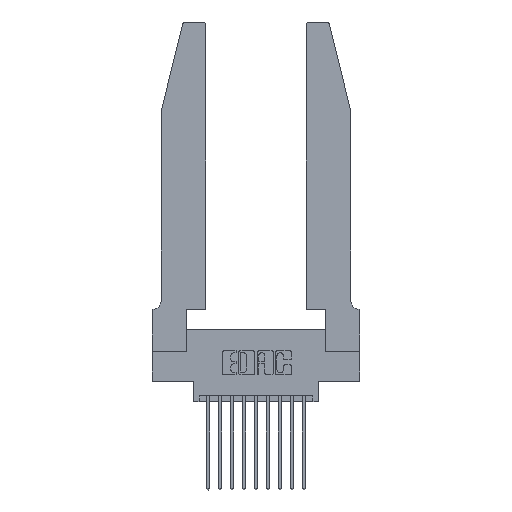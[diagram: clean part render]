
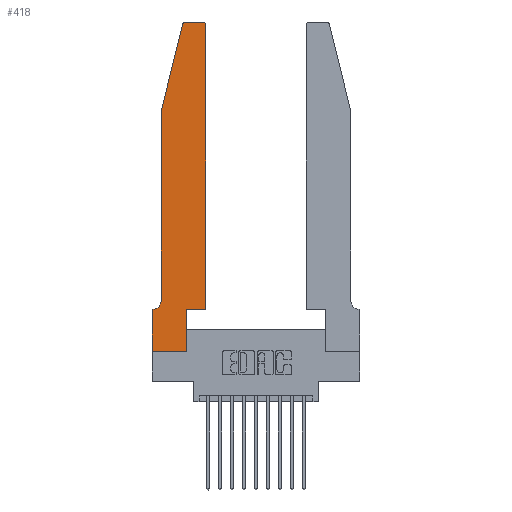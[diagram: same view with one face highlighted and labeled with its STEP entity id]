
A CAD part, top view. The second image highlights one B-rep face of the part: STEP entity #418.
In plain terms, the highlighted planar face has unit normal (0, 0, 1).
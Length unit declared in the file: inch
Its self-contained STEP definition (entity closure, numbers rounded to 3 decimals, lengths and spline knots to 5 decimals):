
#294 = CARTESIAN_POINT ( 'NONE',  ( 0.4505, 0.35, 0.37 ) ) ;
#418 = ADVANCED_FACE ( 'NONE', ( #16232 ), #11630, .T. ) ;
#625 = VERTEX_POINT ( 'NONE', #4278 ) ;
#827 = CARTESIAN_POINT ( 'NONE',  ( 0.4505, 2.72, 0.37 ) ) ;
#834 = CARTESIAN_POINT ( 'NONE',  ( 0., 0., 0.37 ) ) ;
#869 = CIRCLE ( 'NONE', #6204, 0.03 ) ;
#1133 = ORIENTED_EDGE ( 'NONE', *, *, #11162, .T. ) ;
#1213 = VERTEX_POINT ( 'NONE', #11379 ) ;
#1231 = CARTESIAN_POINT ( 'NONE',  ( 0., 0.35, 0.37 ) ) ;
#1258 = VECTOR ( 'NONE', #5156, 39.37008 ) ;
#1449 = EDGE_LOOP ( 'NONE', ( #11076, #2821, #1133, #15777, #2965, #9315, #10290, #14227, #9779, #3927, #10160, #3372 ) ) ;
#1704 = EDGE_CURVE ( 'NONE', #14941, #1213, #3677, .T. ) ;
#1919 = VECTOR ( 'NONE', #13316, 39.37008 ) ;
#2057 = LINE ( 'NONE', #3865, #2455 ) ;
#2366 = LINE ( 'NONE', #13006, #16041 ) ;
#2455 = VECTOR ( 'NONE', #8841, 39.37008 ) ;
#2467 = VECTOR ( 'NONE', #4380, 39.37008 ) ;
#2472 = EDGE_CURVE ( 'NONE', #12306, #9145, #869, .T. ) ;
#2514 = CARTESIAN_POINT ( 'NONE',  ( 0.2605, 2.75, 0.37 ) ) ;
#2601 = DIRECTION ( 'NONE',  ( 1., 0., 0. ) ) ;
#2821 = ORIENTED_EDGE ( 'NONE', *, *, #2472, .T. ) ;
#2903 = CARTESIAN_POINT ( 'NONE',  ( 0.284, 2.72, 0.37 ) ) ;
#2965 = ORIENTED_EDGE ( 'NONE', *, *, #8708, .T. ) ;
#3050 = DIRECTION ( 'NONE',  ( 0., 1., 0. ) ) ;
#3082 = EDGE_CURVE ( 'NONE', #6253, #10421, #6583, .T. ) ;
#3126 = EDGE_CURVE ( 'NONE', #13021, #3900, #12386, .T. ) ;
#3153 = CARTESIAN_POINT ( 'NONE',  ( 0., 0., 0.37 ) ) ;
#3252 = AXIS2_PLACEMENT_3D ( 'NONE', #7584, #15150, #6409 ) ;
#3372 = ORIENTED_EDGE ( 'NONE', *, *, #3082, .T. ) ;
#3518 = EDGE_CURVE ( 'NONE', #10421, #12306, #11980, .T. ) ;
#3677 = LINE ( 'NONE', #5993, #12625 ) ;
#3865 = CARTESIAN_POINT ( 'NONE',  ( 0.0755, 0.35, 0.37 ) ) ;
#3872 = CARTESIAN_POINT ( 'NONE',  ( 0.284, 2.75, 0.37 ) ) ;
#3900 = VERTEX_POINT ( 'NONE', #12139 ) ;
#3927 = ORIENTED_EDGE ( 'NONE', *, *, #1704, .T. ) ;
#4041 = VERTEX_POINT ( 'NONE', #1231 ) ;
#4278 = CARTESIAN_POINT ( 'NONE',  ( 0.0755, 2., 0.37 ) ) ;
#4279 = DIRECTION ( 'NONE',  ( -0.239, -0.971, 0. ) ) ;
#4284 = CARTESIAN_POINT ( 'NONE',  ( 0.0755, 2., 0.37 ) ) ;
#4380 = DIRECTION ( 'NONE',  ( 0., 1., 0. ) ) ;
#4382 = VECTOR ( 'NONE', #4279, 39.37008 ) ;
#4713 = VECTOR ( 'NONE', #15701, 39.37008 ) ;
#5041 = DIRECTION ( 'NONE',  ( 1., 0., 0. ) ) ;
#5156 = DIRECTION ( 'NONE',  ( 1., 0., 0. ) ) ;
#5435 = CIRCLE ( 'NONE', #3252, 0.07 ) ;
#5951 = LINE ( 'NONE', #9512, #4382 ) ;
#5993 = CARTESIAN_POINT ( 'NONE',  ( 0.4505, 0.35, 0.37 ) ) ;
#6204 = AXIS2_PLACEMENT_3D ( 'NONE', #2903, #11786, #15684 ) ;
#6253 = VERTEX_POINT ( 'NONE', #827 ) ;
#6409 = DIRECTION ( 'NONE',  ( -1., 0., 0. ) ) ;
#6479 = CARTESIAN_POINT ( 'NONE',  ( 0., 0., 0.37 ) ) ;
#6532 = CARTESIAN_POINT ( 'NONE',  ( 0., 0.35, 0.37 ) ) ;
#6545 = CARTESIAN_POINT ( 'NONE',  ( 0.25487, 2.72718, 0.37 ) ) ;
#6583 = CIRCLE ( 'NONE', #7807, 0.03 ) ;
#6780 = EDGE_CURVE ( 'NONE', #625, #13459, #9497, .T. ) ;
#7180 = LINE ( 'NONE', #294, #2467 ) ;
#7584 = CARTESIAN_POINT ( 'NONE',  ( 0.0055, 0.42, 0.37 ) ) ;
#7807 = AXIS2_PLACEMENT_3D ( 'NONE', #13849, #9012, #2601 ) ;
#7827 = LINE ( 'NONE', #3153, #1919 ) ;
#7921 = EDGE_CURVE ( 'NONE', #4041, #13021, #7827, .T. ) ;
#8451 = CARTESIAN_POINT ( 'NONE',  ( 0.0755, 0.42, 0.37 ) ) ;
#8708 = EDGE_CURVE ( 'NONE', #13459, #15527, #5435, .T. ) ;
#8789 = CARTESIAN_POINT ( 'NONE',  ( 0.2865, 0.35, 0.37 ) ) ;
#8841 = DIRECTION ( 'NONE',  ( -1., 0., 0. ) ) ;
#9012 = DIRECTION ( 'NONE',  ( 0., 0., 1. ) ) ;
#9115 = DIRECTION ( 'NONE',  ( 0., 0., 1. ) ) ;
#9145 = VERTEX_POINT ( 'NONE', #6545 ) ;
#9315 = ORIENTED_EDGE ( 'NONE', *, *, #9939, .T. ) ;
#9497 = LINE ( 'NONE', #4284, #4713 ) ;
#9512 = CARTESIAN_POINT ( 'NONE',  ( 0.0755, 2., 0.37 ) ) ;
#9566 = EDGE_CURVE ( 'NONE', #1213, #6253, #7180, .T. ) ;
#9779 = ORIENTED_EDGE ( 'NONE', *, *, #13117, .T. ) ;
#9939 = EDGE_CURVE ( 'NONE', #15527, #4041, #2057, .T. ) ;
#10160 = ORIENTED_EDGE ( 'NONE', *, *, #9566, .T. ) ;
#10290 = ORIENTED_EDGE ( 'NONE', *, *, #7921, .T. ) ;
#10421 = VERTEX_POINT ( 'NONE', #15217 ) ;
#10979 = VECTOR ( 'NONE', #15513, 39.37008 ) ;
#11076 = ORIENTED_EDGE ( 'NONE', *, *, #3518, .T. ) ;
#11162 = EDGE_CURVE ( 'NONE', #9145, #625, #5951, .T. ) ;
#11379 = CARTESIAN_POINT ( 'NONE',  ( 0.4505, 0.35, 0.37 ) ) ;
#11630 = PLANE ( 'NONE',  #15953 ) ;
#11786 = DIRECTION ( 'NONE',  ( 0., 0., 1. ) ) ;
#11980 = LINE ( 'NONE', #2514, #10979 ) ;
#12139 = CARTESIAN_POINT ( 'NONE',  ( 0.2865, 0., 0.37 ) ) ;
#12306 = VERTEX_POINT ( 'NONE', #3872 ) ;
#12386 = LINE ( 'NONE', #6479, #1258 ) ;
#12625 = VECTOR ( 'NONE', #5041, 39.37008 ) ;
#12694 = CARTESIAN_POINT ( 'NONE',  ( 0.0055, 0.35, 0.37 ) ) ;
#12914 = DIRECTION ( 'NONE',  ( 1., 0., 0. ) ) ;
#13006 = CARTESIAN_POINT ( 'NONE',  ( 0.2865, 0.35, 0.37 ) ) ;
#13021 = VERTEX_POINT ( 'NONE', #834 ) ;
#13117 = EDGE_CURVE ( 'NONE', #3900, #14941, #2366, .T. ) ;
#13316 = DIRECTION ( 'NONE',  ( 0., -1., 0. ) ) ;
#13459 = VERTEX_POINT ( 'NONE', #8451 ) ;
#13849 = CARTESIAN_POINT ( 'NONE',  ( 0.4205, 2.72, 0.37 ) ) ;
#14227 = ORIENTED_EDGE ( 'NONE', *, *, #3126, .T. ) ;
#14941 = VERTEX_POINT ( 'NONE', #8789 ) ;
#15150 = DIRECTION ( 'NONE',  ( 0., 0., -1. ) ) ;
#15217 = CARTESIAN_POINT ( 'NONE',  ( 0.4205, 2.75, 0.37 ) ) ;
#15513 = DIRECTION ( 'NONE',  ( -1., 0., 0. ) ) ;
#15527 = VERTEX_POINT ( 'NONE', #12694 ) ;
#15684 = DIRECTION ( 'NONE',  ( 1., 0., 0. ) ) ;
#15701 = DIRECTION ( 'NONE',  ( 0., -1., 0. ) ) ;
#15777 = ORIENTED_EDGE ( 'NONE', *, *, #6780, .T. ) ;
#15953 = AXIS2_PLACEMENT_3D ( 'NONE', #6532, #9115, #12914 ) ;
#16041 = VECTOR ( 'NONE', #3050, 39.37008 ) ;
#16232 = FACE_OUTER_BOUND ( 'NONE', #1449, .T. ) ;
